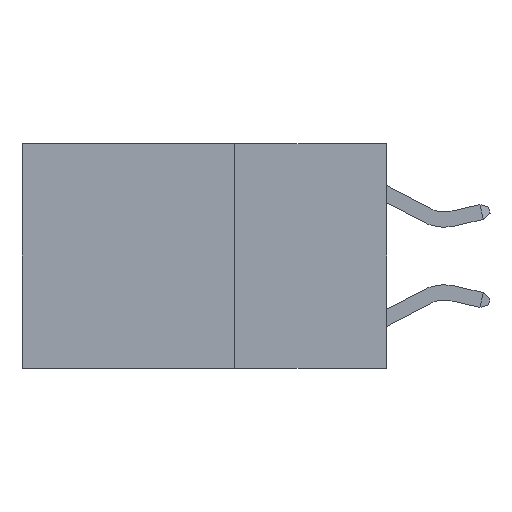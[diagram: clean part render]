
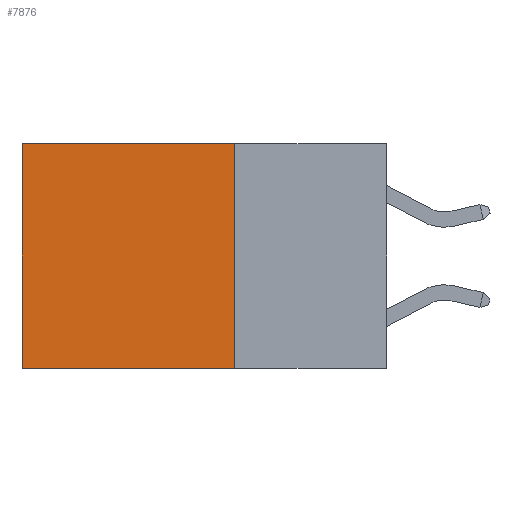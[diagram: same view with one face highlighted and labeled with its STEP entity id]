
A CAD part, left-side view. The second image highlights one B-rep face of the part: STEP entity #7876.
In plain terms, the highlighted planar face has unit normal (-1, 0, 0).
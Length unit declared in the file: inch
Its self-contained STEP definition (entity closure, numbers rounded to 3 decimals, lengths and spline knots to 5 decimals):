
#278 = CARTESIAN_POINT ( 'NONE',  ( 0.2625, 0.6, 0. ) ) ;
#391 = DIRECTION ( 'NONE',  ( 0., 0., -1. ) ) ;
#473 = DIRECTION ( 'NONE',  ( 0., 1., 0. ) ) ;
#808 = DIRECTION ( 'NONE',  ( 0., 1., 0. ) ) ;
#4092 = CARTESIAN_POINT ( 'NONE',  ( 0.2625, 0.25, -0.37 ) ) ;
#4345 = CARTESIAN_POINT ( 'NONE',  ( 0.2625, 0.25, 0. ) ) ;
#4731 = EDGE_CURVE ( 'NONE', #15012, #23478, #16721, .T. ) ;
#4773 = AXIS2_PLACEMENT_3D ( 'NONE', #4845, #28580, #391 ) ;
#4845 = CARTESIAN_POINT ( 'NONE',  ( 0.2625, 0.25, 0. ) ) ;
#6097 = ORIENTED_EDGE ( 'NONE', *, *, #8555, .F. ) ;
#7300 = PLANE ( 'NONE',  #4773 ) ;
#7646 = DIRECTION ( 'NONE',  ( 0., 0., -1. ) ) ;
#7794 = VERTEX_POINT ( 'NONE', #4092 ) ;
#7876 = ADVANCED_FACE ( 'NONE', ( #18647 ), #7300, .F. ) ;
#8555 = EDGE_CURVE ( 'NONE', #7794, #12674, #24550, .T. ) ;
#9894 = CARTESIAN_POINT ( 'NONE',  ( 0.2625, 0.25, 0. ) ) ;
#10797 = VECTOR ( 'NONE', #18595, 39.37008 ) ;
#11315 = ORIENTED_EDGE ( 'NONE', *, *, #29002, .T. ) ;
#12129 = CARTESIAN_POINT ( 'NONE',  ( 0.2625, 0.25, 0. ) ) ;
#12674 = VERTEX_POINT ( 'NONE', #29581 ) ;
#14217 = ORIENTED_EDGE ( 'NONE', *, *, #4731, .T. ) ;
#15012 = VERTEX_POINT ( 'NONE', #9894 ) ;
#16402 = CARTESIAN_POINT ( 'NONE',  ( 0.2625, 0.6, 0. ) ) ;
#16721 = LINE ( 'NONE', #12129, #28987 ) ;
#18595 = DIRECTION ( 'NONE',  ( 0., 0., -1. ) ) ;
#18647 = FACE_OUTER_BOUND ( 'NONE', #23921, .T. ) ;
#23050 = LINE ( 'NONE', #4345, #10797 ) ;
#23478 = VERTEX_POINT ( 'NONE', #278 ) ;
#23892 = LINE ( 'NONE', #16402, #28046 ) ;
#23921 = EDGE_LOOP ( 'NONE', ( #11315, #6097, #25678, #14217 ) ) ;
#24550 = LINE ( 'NONE', #28850, #25376 ) ;
#25376 = VECTOR ( 'NONE', #808, 39.37008 ) ;
#25678 = ORIENTED_EDGE ( 'NONE', *, *, #25859, .F. ) ;
#25859 = EDGE_CURVE ( 'NONE', #15012, #7794, #23050, .T. ) ;
#28046 = VECTOR ( 'NONE', #7646, 39.37008 ) ;
#28580 = DIRECTION ( 'NONE',  ( 1., 0., 0. ) ) ;
#28850 = CARTESIAN_POINT ( 'NONE',  ( 0.2625, 0.25, -0.37 ) ) ;
#28987 = VECTOR ( 'NONE', #473, 39.37008 ) ;
#29002 = EDGE_CURVE ( 'NONE', #23478, #12674, #23892, .T. ) ;
#29581 = CARTESIAN_POINT ( 'NONE',  ( 0.2625, 0.6, -0.37 ) ) ;
